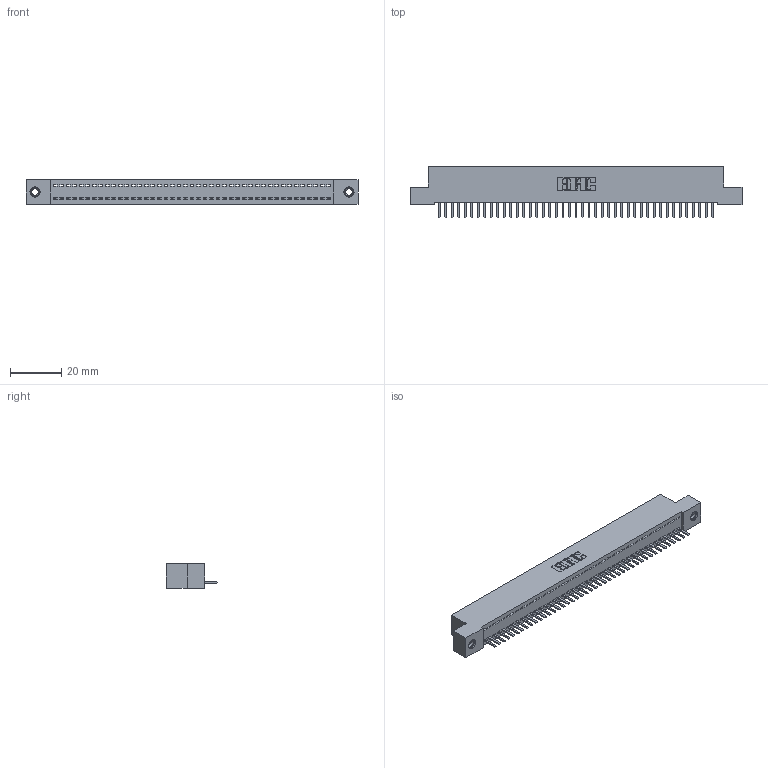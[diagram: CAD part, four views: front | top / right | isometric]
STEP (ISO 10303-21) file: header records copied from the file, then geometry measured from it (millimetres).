
FILE_DESCRIPTION (( 'STEP AP203' ), '1' );
FILE_NAME ('342-043-520-107.STEP', '2018-08-12T13:40:24', ( '' ), ( '' ), 'SwSTEP 2.0', 'SolidWorks 2016', '' );
FILE_SCHEMA (( 'CONFIG_CONTROL_DESIGN' ));
Length unit declared in the file: inch
Products named in the file (4): 342 Part_TI; 345-292-001_345-293-120; 345-250-001_345-250-005-103; 342-043-520-107
Assembly tree (46 placements, depth 2):
  342-043-520-107
    342 Part_TI
    345-292-001_345-293-120  x43
    345-250-001_345-250-005-103  x2
Bounding box: 129.54 x 20.02 x 9.4 mm (x, y, z)
Volume: 11225.4 mm3; surface area: 16139.2 mm2
Topology: 46 solids, 46 shells, 2836 faces, 8347 edges, 5442 vertices
Faces by surface type: plane 1990, cylinder 830, cone 12, torus 4
Entity records: 27326 total; most frequent: CARTESIAN_POINT 4706, ORIENTED_EDGE 4666, DIRECTION 3989, EDGE_CURVE 2333, VECTOR 2181, LINE 2181, VERTEX_POINT 1548, AXIS2_PLACEMENT_3D 904
